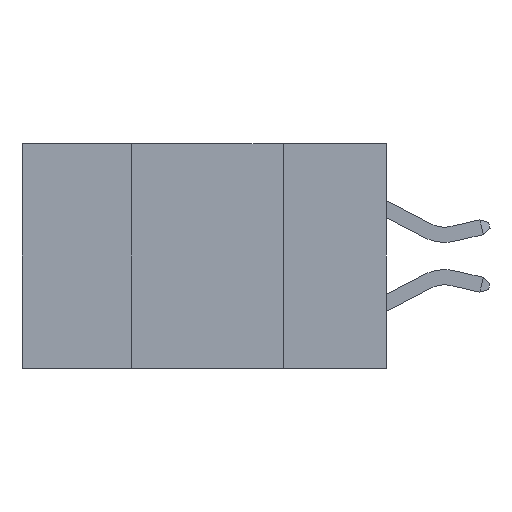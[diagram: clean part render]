
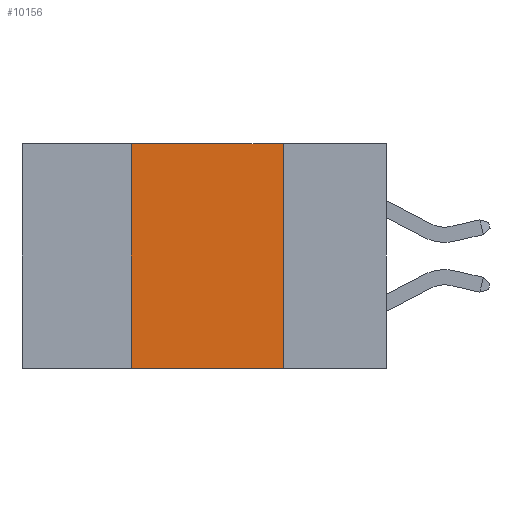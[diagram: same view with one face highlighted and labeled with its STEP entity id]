
A CAD part, left-side view. The second image highlights one B-rep face of the part: STEP entity #10156.
In plain terms, the highlighted planar face has unit normal (-1, 0, 0).
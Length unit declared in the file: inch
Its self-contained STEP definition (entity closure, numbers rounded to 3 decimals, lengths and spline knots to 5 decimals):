
#142 = DIRECTION ( 'NONE',  ( 0., 0., -1. ) ) ;
#327 = VERTEX_POINT ( 'NONE', #941 ) ;
#859 = ORIENTED_EDGE ( 'NONE', *, *, #2541, .F. ) ;
#941 = CARTESIAN_POINT ( 'NONE',  ( 0., 0.42, 0. ) ) ;
#1127 = FACE_OUTER_BOUND ( 'NONE', #3221, .T. ) ;
#1215 = VERTEX_POINT ( 'NONE', #1903 ) ;
#1225 = DIRECTION ( 'NONE',  ( 1., 0., 0. ) ) ;
#1283 = ORIENTED_EDGE ( 'NONE', *, *, #10206, .F. ) ;
#1541 = VECTOR ( 'NONE', #11265, 39.37008 ) ;
#1903 = CARTESIAN_POINT ( 'NONE',  ( 0., 0.17, -0.37 ) ) ;
#2376 = EDGE_CURVE ( 'NONE', #8171, #1215, #10610, .T. ) ;
#2541 = EDGE_CURVE ( 'NONE', #7233, #1215, #3618, .T. ) ;
#2871 = ORIENTED_EDGE ( 'NONE', *, *, #10301, .F. ) ;
#3221 = EDGE_LOOP ( 'NONE', ( #859, #2871, #1283, #3456 ) ) ;
#3456 = ORIENTED_EDGE ( 'NONE', *, *, #2376, .T. ) ;
#3618 = LINE ( 'NONE', #5486, #5336 ) ;
#3770 = CARTESIAN_POINT ( 'NONE',  ( 0., 0.6, 0. ) ) ;
#3821 = CARTESIAN_POINT ( 'NONE',  ( 0., 0.42, -0.37 ) ) ;
#4087 = CARTESIAN_POINT ( 'NONE',  ( 0., 0.6, -0.37 ) ) ;
#4582 = PLANE ( 'NONE',  #10494 ) ;
#5336 = VECTOR ( 'NONE', #142, 39.37008 ) ;
#5486 = CARTESIAN_POINT ( 'NONE',  ( 0., 0.17, -0.37 ) ) ;
#6367 = VECTOR ( 'NONE', #6513, 39.37008 ) ;
#6513 = DIRECTION ( 'NONE',  ( 0., 0., 1. ) ) ;
#7137 = CARTESIAN_POINT ( 'NONE',  ( 0., 0.42, -0.37 ) ) ;
#7233 = VERTEX_POINT ( 'NONE', #11302 ) ;
#8171 = VERTEX_POINT ( 'NONE', #7137 ) ;
#9039 = DIRECTION ( 'NONE',  ( 0., 0., -1. ) ) ;
#10156 = ADVANCED_FACE ( 'NONE', ( #1127 ), #4582, .F. ) ;
#10206 = EDGE_CURVE ( 'NONE', #8171, #327, #10929, .T. ) ;
#10268 = VECTOR ( 'NONE', #11292, 39.37008 ) ;
#10301 = EDGE_CURVE ( 'NONE', #327, #7233, #11352, .T. ) ;
#10494 = AXIS2_PLACEMENT_3D ( 'NONE', #3770, #1225, #9039 ) ;
#10610 = LINE ( 'NONE', #4087, #1541 ) ;
#10929 = LINE ( 'NONE', #3821, #6367 ) ;
#11265 = DIRECTION ( 'NONE',  ( 0., -1., 0. ) ) ;
#11292 = DIRECTION ( 'NONE',  ( 0., -1., 0. ) ) ;
#11302 = CARTESIAN_POINT ( 'NONE',  ( 0., 0.17, 0. ) ) ;
#11352 = LINE ( 'NONE', #11416, #10268 ) ;
#11416 = CARTESIAN_POINT ( 'NONE',  ( 0., 0.6, 0. ) ) ;
